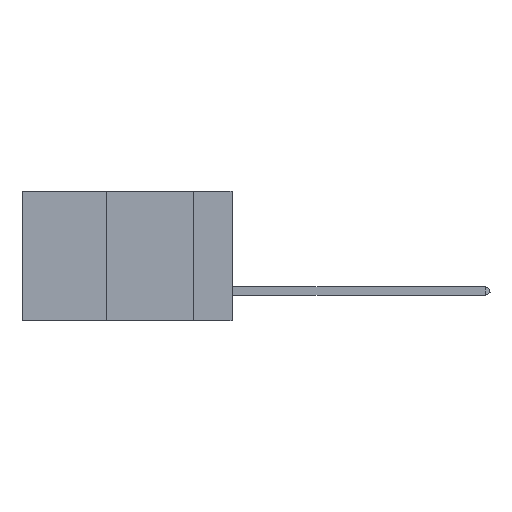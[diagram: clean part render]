
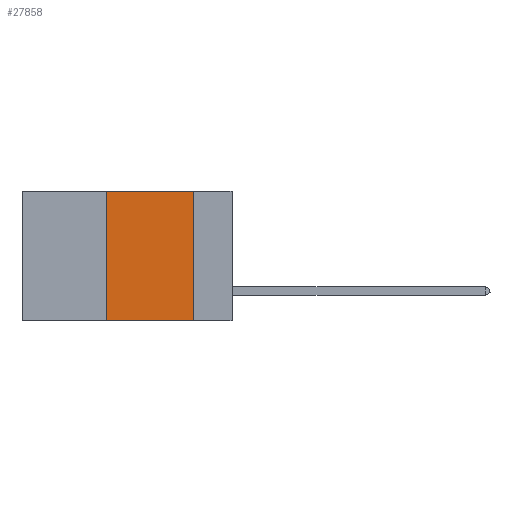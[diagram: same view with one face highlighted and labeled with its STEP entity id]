
A CAD part, left-side view. The second image highlights one B-rep face of the part: STEP entity #27858.
In plain terms, the highlighted planar face has unit normal (-1, 0, 0).
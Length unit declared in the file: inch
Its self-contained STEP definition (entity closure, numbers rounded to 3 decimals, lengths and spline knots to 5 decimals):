
#1306 = ORIENTED_EDGE ( 'NONE', *, *, #5974, .T. ) ;
#2937 = LINE ( 'NONE', #14023, #11963 ) ;
#3206 = EDGE_LOOP ( 'NONE', ( #13696, #14740, #32668, #1306 ) ) ;
#3532 = DIRECTION ( 'NONE',  ( 0., -1., 0. ) ) ;
#4430 = LINE ( 'NONE', #20583, #33503 ) ;
#4789 = CARTESIAN_POINT ( 'NONE',  ( 0., 0.6, 0. ) ) ;
#5974 = EDGE_CURVE ( 'NONE', #14609, #6593, #19694, .T. ) ;
#6593 = VERTEX_POINT ( 'NONE', #25809 ) ;
#7396 = EDGE_CURVE ( 'NONE', #8946, #6593, #4430, .T. ) ;
#8946 = VERTEX_POINT ( 'NONE', #29607 ) ;
#9719 = VECTOR ( 'NONE', #3532, 39.37008 ) ;
#11963 = VECTOR ( 'NONE', #12166, 39.37008 ) ;
#12166 = DIRECTION ( 'NONE',  ( 0., -1., 0. ) ) ;
#13696 = ORIENTED_EDGE ( 'NONE', *, *, #7396, .F. ) ;
#13914 = CARTESIAN_POINT ( 'NONE',  ( 0., 0.6, -0.37 ) ) ;
#14023 = CARTESIAN_POINT ( 'NONE',  ( 0., 0.6, 0. ) ) ;
#14609 = VERTEX_POINT ( 'NONE', #21749 ) ;
#14740 = ORIENTED_EDGE ( 'NONE', *, *, #30285, .F. ) ;
#15556 = DIRECTION ( 'NONE',  ( 0., 0., 1. ) ) ;
#15692 = DIRECTION ( 'NONE',  ( 0., 0., -1. ) ) ;
#16430 = EDGE_CURVE ( 'NONE', #14609, #26215, #18278, .T. ) ;
#18096 = CARTESIAN_POINT ( 'NONE',  ( 0., 0.36, 0. ) ) ;
#18278 = LINE ( 'NONE', #18096, #30985 ) ;
#18408 = DIRECTION ( 'NONE',  ( 0., 0., -1. ) ) ;
#19694 = LINE ( 'NONE', #13914, #9719 ) ;
#20583 = CARTESIAN_POINT ( 'NONE',  ( 0., 0.11, 0. ) ) ;
#21749 = CARTESIAN_POINT ( 'NONE',  ( 0., 0.36, -0.37 ) ) ;
#22472 = CARTESIAN_POINT ( 'NONE',  ( 0., 0.36, 0. ) ) ;
#23847 = PLANE ( 'NONE',  #25658 ) ;
#24395 = DIRECTION ( 'NONE',  ( 1., 0., 0. ) ) ;
#25658 = AXIS2_PLACEMENT_3D ( 'NONE', #4789, #24395, #15692 ) ;
#25809 = CARTESIAN_POINT ( 'NONE',  ( 0., 0.11, -0.37 ) ) ;
#26215 = VERTEX_POINT ( 'NONE', #22472 ) ;
#27116 = FACE_OUTER_BOUND ( 'NONE', #3206, .T. ) ;
#27858 = ADVANCED_FACE ( 'NONE', ( #27116 ), #23847, .F. ) ;
#29607 = CARTESIAN_POINT ( 'NONE',  ( 0., 0.11, 0. ) ) ;
#30285 = EDGE_CURVE ( 'NONE', #26215, #8946, #2937, .T. ) ;
#30985 = VECTOR ( 'NONE', #15556, 39.37008 ) ;
#32668 = ORIENTED_EDGE ( 'NONE', *, *, #16430, .F. ) ;
#33503 = VECTOR ( 'NONE', #18408, 39.37008 ) ;
